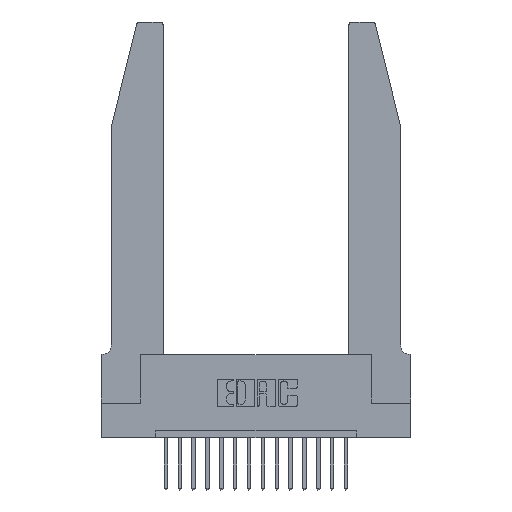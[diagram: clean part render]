
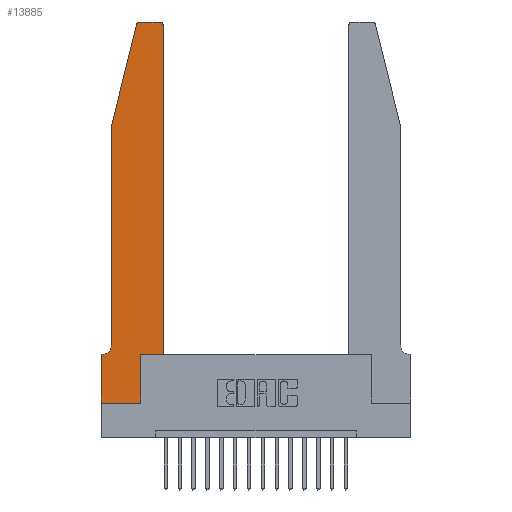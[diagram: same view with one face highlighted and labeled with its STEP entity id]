
A CAD part, top view. The second image highlights one B-rep face of the part: STEP entity #13885.
In plain terms, the highlighted planar face has unit normal (0, 0, 1).
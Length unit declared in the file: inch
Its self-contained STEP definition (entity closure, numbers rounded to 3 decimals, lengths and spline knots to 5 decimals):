
#88 = ORIENTED_EDGE ( 'NONE', *, *, #10458, .T. ) ;
#384 = LINE ( 'NONE', #11978, #7064 ) ;
#386 = EDGE_CURVE ( 'NONE', #7913, #17544, #11872, .T. ) ;
#512 = PLANE ( 'NONE',  #13194 ) ;
#556 = CARTESIAN_POINT ( 'NONE',  ( 0.4505, 0.35, 0.37 ) ) ;
#618 = EDGE_CURVE ( 'NONE', #14619, #9750, #12782, .T. ) ;
#1554 = DIRECTION ( 'NONE',  ( -1., 0., 0. ) ) ;
#1660 = DIRECTION ( 'NONE',  ( 1., 0., 0. ) ) ;
#1748 = CARTESIAN_POINT ( 'NONE',  ( 0., 0.35, 0.37 ) ) ;
#1810 = VERTEX_POINT ( 'NONE', #2043 ) ;
#1814 = ORIENTED_EDGE ( 'NONE', *, *, #7897, .T. ) ;
#2043 = CARTESIAN_POINT ( 'NONE',  ( 0.0755, 2., 0.37 ) ) ;
#2114 = VECTOR ( 'NONE', #6960, 39.37008 ) ;
#2186 = VECTOR ( 'NONE', #16632, 39.37008 ) ;
#2378 = DIRECTION ( 'NONE',  ( 0., -1., 0. ) ) ;
#2392 = CARTESIAN_POINT ( 'NONE',  ( 0.25487, 2.72718, 0.37 ) ) ;
#2639 = CARTESIAN_POINT ( 'NONE',  ( 0., 0., 0.37 ) ) ;
#2674 = CARTESIAN_POINT ( 'NONE',  ( 0.0755, 0.35, 0.37 ) ) ;
#2676 = EDGE_LOOP ( 'NONE', ( #2792, #10016, #88, #4322, #5467, #1814, #12960, #10738, #16864, #18624, #14216, #2691 ) ) ;
#2691 = ORIENTED_EDGE ( 'NONE', *, *, #9665, .T. ) ;
#2792 = ORIENTED_EDGE ( 'NONE', *, *, #3284, .T. ) ;
#2967 = VECTOR ( 'NONE', #2378, 39.37008 ) ;
#3207 = CARTESIAN_POINT ( 'NONE',  ( 0.4205, 2.75, 0.37 ) ) ;
#3284 = EDGE_CURVE ( 'NONE', #18999, #16972, #16485, .T. ) ;
#3440 = VERTEX_POINT ( 'NONE', #8487 ) ;
#3536 = EDGE_CURVE ( 'NONE', #18292, #18796, #6560, .T. ) ;
#3674 = LINE ( 'NONE', #4064, #14964 ) ;
#3839 = VECTOR ( 'NONE', #1554, 39.37008 ) ;
#4064 = CARTESIAN_POINT ( 'NONE',  ( 0., 0., 0.37 ) ) ;
#4322 = ORIENTED_EDGE ( 'NONE', *, *, #9688, .T. ) ;
#4768 = DIRECTION ( 'NONE',  ( 0., 0., -1. ) ) ;
#4828 = CARTESIAN_POINT ( 'NONE',  ( 0.0055, 0.42, 0.37 ) ) ;
#4876 = EDGE_CURVE ( 'NONE', #3440, #14619, #15520, .T. ) ;
#4947 = LINE ( 'NONE', #6847, #10013 ) ;
#5023 = CARTESIAN_POINT ( 'NONE',  ( 0., 0.35, 0.37 ) ) ;
#5124 = FACE_OUTER_BOUND ( 'NONE', #2676, .T. ) ;
#5467 = ORIENTED_EDGE ( 'NONE', *, *, #386, .T. ) ;
#5571 = DIRECTION ( 'NONE',  ( 0., 1., 0. ) ) ;
#6516 = VERTEX_POINT ( 'NONE', #2392 ) ;
#6560 = LINE ( 'NONE', #2639, #13504 ) ;
#6847 = CARTESIAN_POINT ( 'NONE',  ( 0.4505, 0.35, 0.37 ) ) ;
#6960 = DIRECTION ( 'NONE',  ( -1., 0., 0. ) ) ;
#7041 = CARTESIAN_POINT ( 'NONE',  ( 0.2865, 0.35, 0.37 ) ) ;
#7064 = VECTOR ( 'NONE', #12159, 39.37008 ) ;
#7442 = AXIS2_PLACEMENT_3D ( 'NONE', #14158, #17111, #15758 ) ;
#7673 = DIRECTION ( 'NONE',  ( 0., 0., 1. ) ) ;
#7897 = EDGE_CURVE ( 'NONE', #17544, #18292, #17318, .T. ) ;
#7913 = VERTEX_POINT ( 'NONE', #9850 ) ;
#8103 = CARTESIAN_POINT ( 'NONE',  ( 0.0755, 2., 0.37 ) ) ;
#8144 = VECTOR ( 'NONE', #15877, 39.37008 ) ;
#8253 = LINE ( 'NONE', #8103, #2967 ) ;
#8487 = CARTESIAN_POINT ( 'NONE',  ( 0.2865, 0., 0.37 ) ) ;
#8672 = CARTESIAN_POINT ( 'NONE',  ( 0., 0., 0.37 ) ) ;
#8691 = EDGE_CURVE ( 'NONE', #16972, #6516, #13833, .T. ) ;
#9006 = AXIS2_PLACEMENT_3D ( 'NONE', #16181, #7673, #13495 ) ;
#9093 = DIRECTION ( 'NONE',  ( -1., 0., 0. ) ) ;
#9362 = EDGE_CURVE ( 'NONE', #18796, #3440, #3674, .T. ) ;
#9415 = CIRCLE ( 'NONE', #7442, 0.03 ) ;
#9665 = EDGE_CURVE ( 'NONE', #15038, #18999, #9415, .T. ) ;
#9688 = EDGE_CURVE ( 'NONE', #1810, #7913, #8253, .T. ) ;
#9750 = VERTEX_POINT ( 'NONE', #15101 ) ;
#9850 = CARTESIAN_POINT ( 'NONE',  ( 0.0755, 0.42, 0.37 ) ) ;
#10013 = VECTOR ( 'NONE', #5571, 39.37008 ) ;
#10016 = ORIENTED_EDGE ( 'NONE', *, *, #8691, .T. ) ;
#10042 = CARTESIAN_POINT ( 'NONE',  ( 0.0055, 0.35, 0.37 ) ) ;
#10343 = CARTESIAN_POINT ( 'NONE',  ( 0.2605, 2.75, 0.37 ) ) ;
#10458 = EDGE_CURVE ( 'NONE', #6516, #1810, #384, .T. ) ;
#10738 = ORIENTED_EDGE ( 'NONE', *, *, #9362, .T. ) ;
#10800 = DIRECTION ( 'NONE',  ( 0., 0., 1. ) ) ;
#11240 = AXIS2_PLACEMENT_3D ( 'NONE', #4828, #4768, #9093 ) ;
#11553 = EDGE_CURVE ( 'NONE', #9750, #15038, #4947, .T. ) ;
#11570 = CARTESIAN_POINT ( 'NONE',  ( 0.2865, 0.35, 0.37 ) ) ;
#11872 = CIRCLE ( 'NONE', #11240, 0.07 ) ;
#11978 = CARTESIAN_POINT ( 'NONE',  ( 0.0755, 2., 0.37 ) ) ;
#12159 = DIRECTION ( 'NONE',  ( -0.239, -0.971, 0. ) ) ;
#12494 = DIRECTION ( 'NONE',  ( 1., 0., 0. ) ) ;
#12782 = LINE ( 'NONE', #556, #2186 ) ;
#12960 = ORIENTED_EDGE ( 'NONE', *, *, #3536, .T. ) ;
#13194 = AXIS2_PLACEMENT_3D ( 'NONE', #5023, #10800, #12494 ) ;
#13495 = DIRECTION ( 'NONE',  ( 1., 0., 0. ) ) ;
#13504 = VECTOR ( 'NONE', #18861, 39.37008 ) ;
#13833 = CIRCLE ( 'NONE', #9006, 0.03 ) ;
#13885 = ADVANCED_FACE ( 'NONE', ( #5124 ), #512, .T. ) ;
#13928 = CARTESIAN_POINT ( 'NONE',  ( 0.4505, 2.72, 0.37 ) ) ;
#14158 = CARTESIAN_POINT ( 'NONE',  ( 0.4205, 2.72, 0.37 ) ) ;
#14216 = ORIENTED_EDGE ( 'NONE', *, *, #11553, .T. ) ;
#14619 = VERTEX_POINT ( 'NONE', #7041 ) ;
#14964 = VECTOR ( 'NONE', #1660, 39.37008 ) ;
#15038 = VERTEX_POINT ( 'NONE', #13928 ) ;
#15101 = CARTESIAN_POINT ( 'NONE',  ( 0.4505, 0.35, 0.37 ) ) ;
#15520 = LINE ( 'NONE', #11570, #8144 ) ;
#15758 = DIRECTION ( 'NONE',  ( 1., 0., 0. ) ) ;
#15877 = DIRECTION ( 'NONE',  ( 0., 1., 0. ) ) ;
#16181 = CARTESIAN_POINT ( 'NONE',  ( 0.284, 2.72, 0.37 ) ) ;
#16485 = LINE ( 'NONE', #10343, #3839 ) ;
#16632 = DIRECTION ( 'NONE',  ( 1., 0., 0. ) ) ;
#16864 = ORIENTED_EDGE ( 'NONE', *, *, #4876, .T. ) ;
#16972 = VERTEX_POINT ( 'NONE', #18672 ) ;
#17111 = DIRECTION ( 'NONE',  ( 0., 0., 1. ) ) ;
#17318 = LINE ( 'NONE', #2674, #2114 ) ;
#17544 = VERTEX_POINT ( 'NONE', #10042 ) ;
#18292 = VERTEX_POINT ( 'NONE', #1748 ) ;
#18624 = ORIENTED_EDGE ( 'NONE', *, *, #618, .T. ) ;
#18672 = CARTESIAN_POINT ( 'NONE',  ( 0.284, 2.75, 0.37 ) ) ;
#18796 = VERTEX_POINT ( 'NONE', #8672 ) ;
#18861 = DIRECTION ( 'NONE',  ( 0., -1., 0. ) ) ;
#18999 = VERTEX_POINT ( 'NONE', #3207 ) ;
